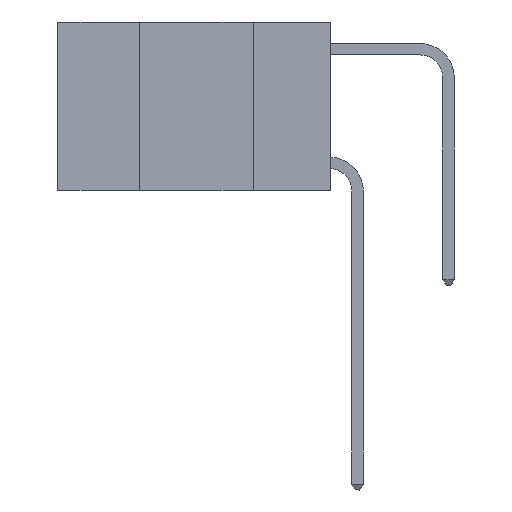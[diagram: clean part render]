
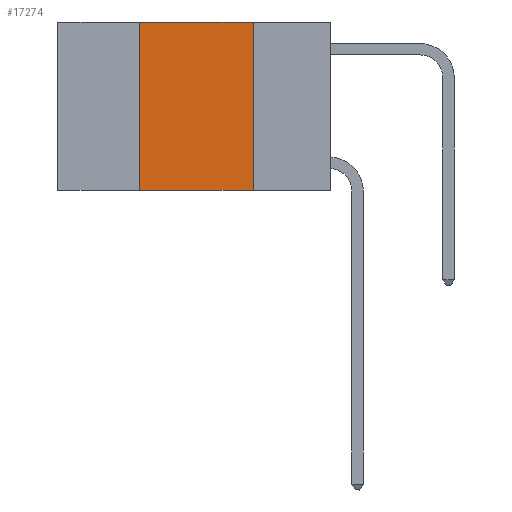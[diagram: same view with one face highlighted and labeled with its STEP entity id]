
A CAD part, left-side view. The second image highlights one B-rep face of the part: STEP entity #17274.
In plain terms, the highlighted planar face has unit normal (-1, 0, 0).
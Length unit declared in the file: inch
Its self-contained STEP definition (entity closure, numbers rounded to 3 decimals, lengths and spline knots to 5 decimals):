
#326 = VECTOR ( 'NONE', #751, 39.37008 ) ;
#688 = CARTESIAN_POINT ( 'NONE',  ( 0., 0.17, 0. ) ) ;
#751 = DIRECTION ( 'NONE',  ( 0., 0., -1. ) ) ;
#834 = AXIS2_PLACEMENT_3D ( 'NONE', #10229, #11590, #3545 ) ;
#1673 = ORIENTED_EDGE ( 'NONE', *, *, #7861, .F. ) ;
#1973 = LINE ( 'NONE', #10149, #9966 ) ;
#3506 = LINE ( 'NONE', #11656, #17354 ) ;
#3545 = DIRECTION ( 'NONE',  ( 0., 0., -1. ) ) ;
#3607 = VERTEX_POINT ( 'NONE', #14456 ) ;
#4433 = EDGE_CURVE ( 'NONE', #15170, #3607, #3506, .T. ) ;
#5076 = CARTESIAN_POINT ( 'NONE',  ( 0., 0.6, -0.37 ) ) ;
#5747 = CARTESIAN_POINT ( 'NONE',  ( 0., 0.17, -0.37 ) ) ;
#7593 = VERTEX_POINT ( 'NONE', #13185 ) ;
#7624 = PLANE ( 'NONE',  #834 ) ;
#7861 = EDGE_CURVE ( 'NONE', #7593, #15170, #1973, .T. ) ;
#8112 = ORIENTED_EDGE ( 'NONE', *, *, #4433, .F. ) ;
#8257 = VECTOR ( 'NONE', #9105, 39.37008 ) ;
#9086 = DIRECTION ( 'NONE',  ( 0., -1., 0. ) ) ;
#9097 = EDGE_LOOP ( 'NONE', ( #14970, #8112, #1673, #9215 ) ) ;
#9103 = EDGE_CURVE ( 'NONE', #7593, #16495, #15188, .T. ) ;
#9105 = DIRECTION ( 'NONE',  ( 0., -1., 0. ) ) ;
#9215 = ORIENTED_EDGE ( 'NONE', *, *, #9103, .T. ) ;
#9966 = VECTOR ( 'NONE', #12572, 39.37008 ) ;
#10149 = CARTESIAN_POINT ( 'NONE',  ( 0., 0.42, 0. ) ) ;
#10229 = CARTESIAN_POINT ( 'NONE',  ( 0., 0.6, 0. ) ) ;
#10965 = CARTESIAN_POINT ( 'NONE',  ( 0., 0.42, 0. ) ) ;
#11590 = DIRECTION ( 'NONE',  ( 1., 0., 0. ) ) ;
#11656 = CARTESIAN_POINT ( 'NONE',  ( 0., 0.6, 0. ) ) ;
#12572 = DIRECTION ( 'NONE',  ( 0., 0., 1. ) ) ;
#13185 = CARTESIAN_POINT ( 'NONE',  ( 0., 0.42, -0.37 ) ) ;
#14456 = CARTESIAN_POINT ( 'NONE',  ( 0., 0.17, 0. ) ) ;
#14811 = FACE_OUTER_BOUND ( 'NONE', #9097, .T. ) ;
#14970 = ORIENTED_EDGE ( 'NONE', *, *, #15346, .F. ) ;
#15170 = VERTEX_POINT ( 'NONE', #10965 ) ;
#15188 = LINE ( 'NONE', #5076, #8257 ) ;
#15346 = EDGE_CURVE ( 'NONE', #3607, #16495, #16114, .T. ) ;
#16114 = LINE ( 'NONE', #688, #326 ) ;
#16495 = VERTEX_POINT ( 'NONE', #5747 ) ;
#17274 = ADVANCED_FACE ( 'NONE', ( #14811 ), #7624, .F. ) ;
#17354 = VECTOR ( 'NONE', #9086, 39.37008 ) ;
